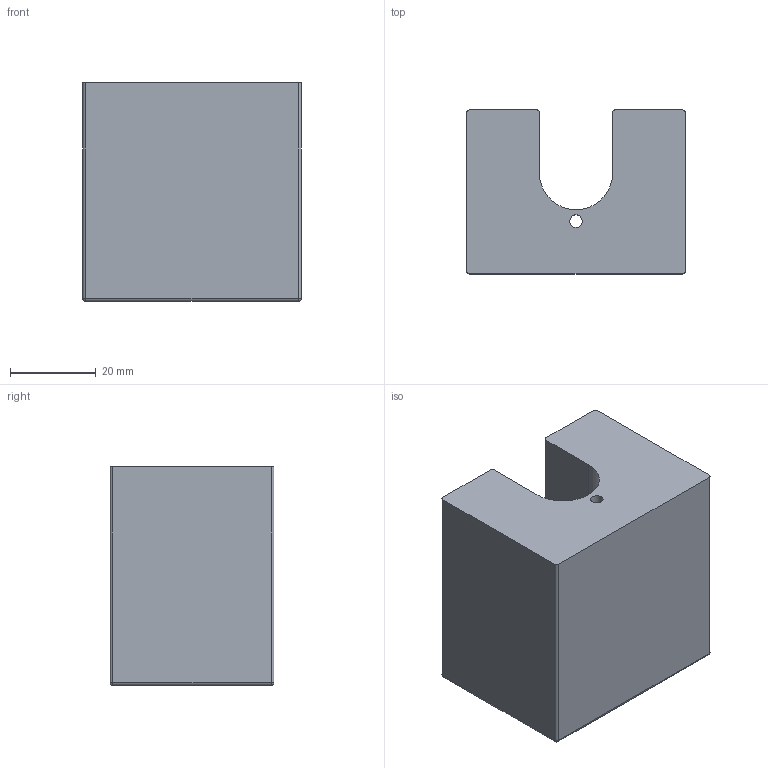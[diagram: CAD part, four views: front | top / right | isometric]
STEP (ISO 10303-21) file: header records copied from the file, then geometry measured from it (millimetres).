
FILE_DESCRIPTION(/* description */ (''),/* implementation_level */ '2;1');
FILE_NAME(/* name */ 'Jig 4.stp',/* time_stamp */ '2019-03-23T15:17:22-05:00',/* author */ ('johne'),/* organization */ (''),/* preprocessor_version */ 'ST-DEVELOPER v16.13',/* originating_system */ 'Autodesk Inventor 2018',/* authorisation */ '');
FILE_SCHEMA (('AUTOMOTIVE_DESIGN { 1 0 10303 214 3 1 1 }'));
Length unit declared in the file: inch
Products named in the file (1): Jig 4
Bounding box: 50.8 x 38.1 x 50.8 mm (x, y, z)
Volume: 71004 mm3; surface area: 15295.3 mm2
Topology: 1 solids, 1 shells, 74 faces, 173 edges, 103 vertices
Faces by surface type: plane 34, cylinder 29, sphere 8, torus 3
Full cylindrical faces by diameter (mm): 2.921 x1
Entity records: 2149 total; most frequent: CARTESIAN_POINT 396, DIRECTION 368, ORIENTED_EDGE 344, EDGE_CURVE 172, AXIS2_PLACEMENT_3D 125, LINE 118, VECTOR 118, VERTEX_POINT 103
